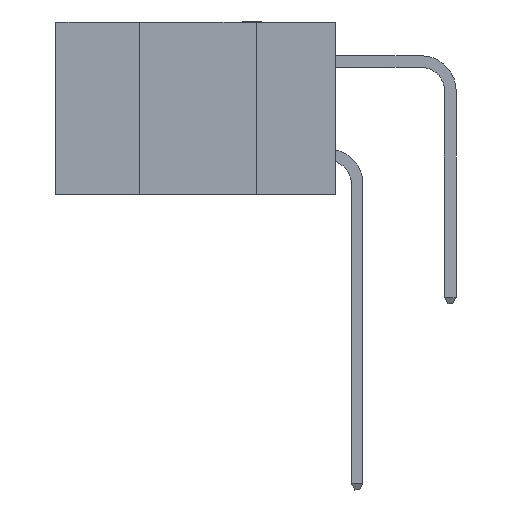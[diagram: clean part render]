
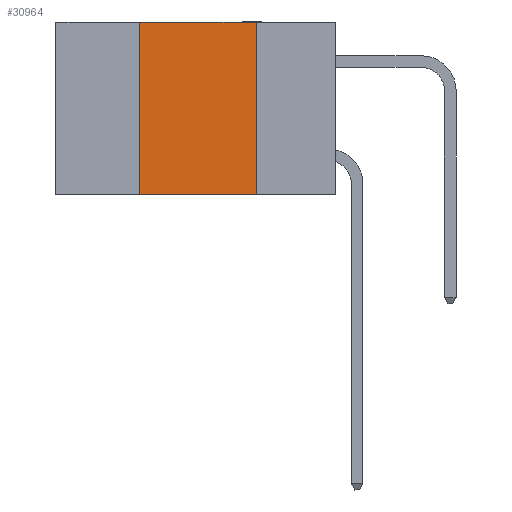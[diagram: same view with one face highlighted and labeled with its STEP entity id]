
A CAD part, left-side view. The second image highlights one B-rep face of the part: STEP entity #30964.
In plain terms, the highlighted planar face has unit normal (-1, 0, 0).
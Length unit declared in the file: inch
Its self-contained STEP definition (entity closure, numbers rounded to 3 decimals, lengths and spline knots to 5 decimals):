
#1104 = DIRECTION ( 'NONE',  ( 0., -1., 0. ) ) ;
#2495 = AXIS2_PLACEMENT_3D ( 'NONE', #25480, #15844, #5919 ) ;
#3369 = CARTESIAN_POINT ( 'NONE',  ( 0., 0.42, 0. ) ) ;
#3796 = VERTEX_POINT ( 'NONE', #18099 ) ;
#5006 = LINE ( 'NONE', #15219, #9078 ) ;
#5398 = LINE ( 'NONE', #30154, #23129 ) ;
#5919 = DIRECTION ( 'NONE',  ( 0., 0., -1. ) ) ;
#9078 = VECTOR ( 'NONE', #18449, 39.37008 ) ;
#9486 = DIRECTION ( 'NONE',  ( 0., 0., 1. ) ) ;
#9537 = CARTESIAN_POINT ( 'NONE',  ( 0., 0.17, 0. ) ) ;
#9942 = VERTEX_POINT ( 'NONE', #9537 ) ;
#11656 = CARTESIAN_POINT ( 'NONE',  ( 0., 0.17, -0.37 ) ) ;
#12048 = EDGE_CURVE ( 'NONE', #23705, #3796, #36383, .T. ) ;
#13043 = EDGE_CURVE ( 'NONE', #3796, #9942, #5398, .T. ) ;
#13812 = VECTOR ( 'NONE', #20968, 39.37008 ) ;
#15219 = CARTESIAN_POINT ( 'NONE',  ( 0., 0.17, 0. ) ) ;
#15550 = PLANE ( 'NONE',  #2495 ) ;
#15844 = DIRECTION ( 'NONE',  ( 1., 0., 0. ) ) ;
#16454 = EDGE_CURVE ( 'NONE', #23705, #33301, #25495, .T. ) ;
#17754 = CARTESIAN_POINT ( 'NONE',  ( 0., 0.42, -0.37 ) ) ;
#18099 = CARTESIAN_POINT ( 'NONE',  ( 0., 0.42, 0. ) ) ;
#18449 = DIRECTION ( 'NONE',  ( 0., 0., -1. ) ) ;
#18928 = FACE_OUTER_BOUND ( 'NONE', #31121, .T. ) ;
#20968 = DIRECTION ( 'NONE',  ( 0., -1., 0. ) ) ;
#21275 = ORIENTED_EDGE ( 'NONE', *, *, #12048, .F. ) ;
#23129 = VECTOR ( 'NONE', #1104, 39.37008 ) ;
#23362 = ORIENTED_EDGE ( 'NONE', *, *, #13043, .F. ) ;
#23705 = VERTEX_POINT ( 'NONE', #17754 ) ;
#24252 = ORIENTED_EDGE ( 'NONE', *, *, #16454, .T. ) ;
#24451 = ORIENTED_EDGE ( 'NONE', *, *, #34121, .F. ) ;
#25480 = CARTESIAN_POINT ( 'NONE',  ( 0., 0.6, 0. ) ) ;
#25495 = LINE ( 'NONE', #40917, #13812 ) ;
#28833 = VECTOR ( 'NONE', #9486, 39.37008 ) ;
#30154 = CARTESIAN_POINT ( 'NONE',  ( 0., 0.6, 0. ) ) ;
#30964 = ADVANCED_FACE ( 'NONE', ( #18928 ), #15550, .F. ) ;
#31121 = EDGE_LOOP ( 'NONE', ( #24451, #23362, #21275, #24252 ) ) ;
#33301 = VERTEX_POINT ( 'NONE', #11656 ) ;
#34121 = EDGE_CURVE ( 'NONE', #9942, #33301, #5006, .T. ) ;
#36383 = LINE ( 'NONE', #3369, #28833 ) ;
#40917 = CARTESIAN_POINT ( 'NONE',  ( 0., 0.6, -0.37 ) ) ;
